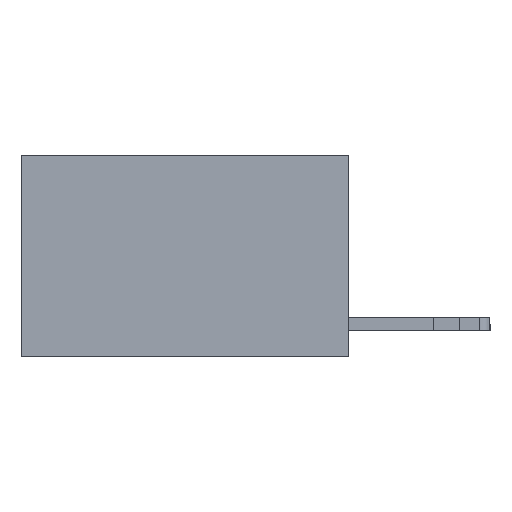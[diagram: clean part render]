
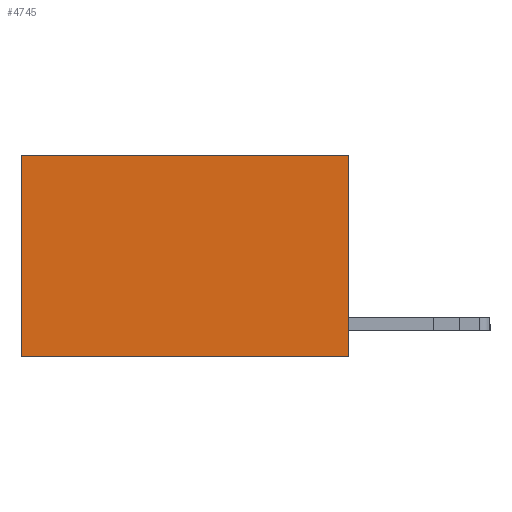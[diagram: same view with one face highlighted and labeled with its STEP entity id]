
A CAD part, left-side view. The second image highlights one B-rep face of the part: STEP entity #4745.
In plain terms, the highlighted planar face has unit normal (-1, 0, 0).
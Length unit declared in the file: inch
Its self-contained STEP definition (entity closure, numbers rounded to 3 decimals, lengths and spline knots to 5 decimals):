
#260 = DIRECTION ( 'NONE',  ( 1., 0., 0. ) ) ;
#1275 = LINE ( 'NONE', #4707, #2811 ) ;
#1282 = EDGE_CURVE ( 'NONE', #2066, #9935, #9819, .T. ) ;
#1503 = VERTEX_POINT ( 'NONE', #12393 ) ;
#1532 = ORIENTED_EDGE ( 'NONE', *, *, #5991, .T. ) ;
#2066 = VERTEX_POINT ( 'NONE', #4483 ) ;
#2213 = AXIS2_PLACEMENT_3D ( 'NONE', #3753, #260, #8396 ) ;
#2459 = PLANE ( 'NONE',  #2213 ) ;
#2811 = VECTOR ( 'NONE', #8278, 39.37008 ) ;
#2917 = ORIENTED_EDGE ( 'NONE', *, *, #12118, .T. ) ;
#3753 = CARTESIAN_POINT ( 'NONE',  ( 0.2625, 0., 0. ) ) ;
#4057 = EDGE_LOOP ( 'NONE', ( #1532, #9291, #8545, #2917 ) ) ;
#4483 = CARTESIAN_POINT ( 'NONE',  ( 0.2625, 0., 0. ) ) ;
#4707 = CARTESIAN_POINT ( 'NONE',  ( 0.2625, 0., 0. ) ) ;
#4745 = ADVANCED_FACE ( 'NONE', ( #14181 ), #2459, .F. ) ;
#5828 = LINE ( 'NONE', #12659, #9185 ) ;
#5991 = EDGE_CURVE ( 'NONE', #1503, #9943, #10679, .T. ) ;
#6259 = CARTESIAN_POINT ( 'NONE',  ( 0.2625, 0.6, 0. ) ) ;
#7080 = CARTESIAN_POINT ( 'NONE',  ( 0.2625, 0., -0.37 ) ) ;
#7979 = VECTOR ( 'NONE', #14339, 39.37008 ) ;
#8278 = DIRECTION ( 'NONE',  ( 0., 1., 0. ) ) ;
#8396 = DIRECTION ( 'NONE',  ( 0., 0., -1. ) ) ;
#8545 = ORIENTED_EDGE ( 'NONE', *, *, #1282, .F. ) ;
#9185 = VECTOR ( 'NONE', #11606, 39.37008 ) ;
#9291 = ORIENTED_EDGE ( 'NONE', *, *, #13597, .F. ) ;
#9819 = LINE ( 'NONE', #12163, #12188 ) ;
#9935 = VERTEX_POINT ( 'NONE', #7080 ) ;
#9943 = VERTEX_POINT ( 'NONE', #11563 ) ;
#10679 = LINE ( 'NONE', #6259, #7979 ) ;
#10738 = DIRECTION ( 'NONE',  ( 0., 0., -1. ) ) ;
#11563 = CARTESIAN_POINT ( 'NONE',  ( 0.2625, 0.6, -0.37 ) ) ;
#11606 = DIRECTION ( 'NONE',  ( 0., 1., 0. ) ) ;
#12118 = EDGE_CURVE ( 'NONE', #2066, #1503, #1275, .T. ) ;
#12163 = CARTESIAN_POINT ( 'NONE',  ( 0.2625, 0., 0. ) ) ;
#12188 = VECTOR ( 'NONE', #10738, 39.37008 ) ;
#12393 = CARTESIAN_POINT ( 'NONE',  ( 0.2625, 0.6, 0. ) ) ;
#12659 = CARTESIAN_POINT ( 'NONE',  ( 0.2625, 0., -0.37 ) ) ;
#13597 = EDGE_CURVE ( 'NONE', #9935, #9943, #5828, .T. ) ;
#14181 = FACE_OUTER_BOUND ( 'NONE', #4057, .T. ) ;
#14339 = DIRECTION ( 'NONE',  ( 0., 0., -1. ) ) ;
